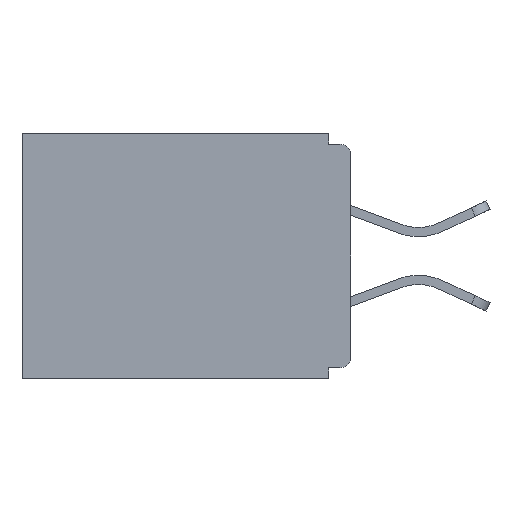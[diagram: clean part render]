
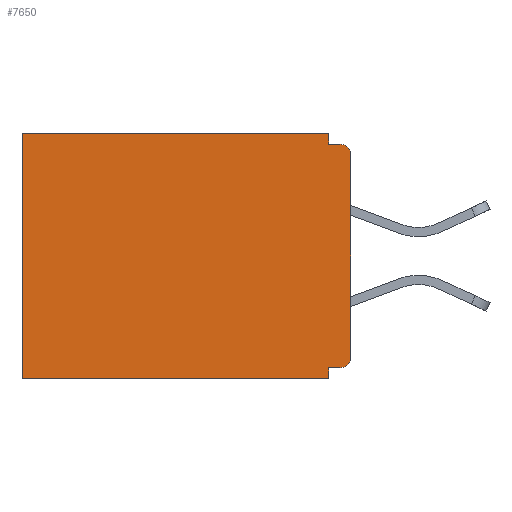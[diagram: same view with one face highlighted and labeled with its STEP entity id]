
A CAD part, left-side view. The second image highlights one B-rep face of the part: STEP entity #7650.
In plain terms, the highlighted planar face has unit normal (-1, 0, 0).
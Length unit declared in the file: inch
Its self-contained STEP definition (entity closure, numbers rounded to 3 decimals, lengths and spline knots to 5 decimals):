
#247 = EDGE_CURVE ( 'NONE', #10702, #9965, #11336, .T. ) ;
#285 = CIRCLE ( 'NONE', #10075, 0.015 ) ;
#392 = ORIENTED_EDGE ( 'NONE', *, *, #9194, .T. ) ;
#586 = VECTOR ( 'NONE', #7604, 39.37008 ) ;
#631 = VERTEX_POINT ( 'NONE', #12298 ) ;
#679 = DIRECTION ( 'NONE',  ( -1., 0., 0. ) ) ;
#1285 = CARTESIAN_POINT ( 'NONE',  ( 0.298, 0., 0. ) ) ;
#1431 = VERTEX_POINT ( 'NONE', #9696 ) ;
#1735 = CARTESIAN_POINT ( 'NONE',  ( 0.298, 0.031, -0.343 ) ) ;
#1775 = VECTOR ( 'NONE', #13323, 39.37008 ) ;
#1969 = PLANE ( 'NONE',  #9557 ) ;
#1972 = DIRECTION ( 'NONE',  ( 0., 0., -1. ) ) ;
#2337 = LINE ( 'NONE', #13573, #7540 ) ;
#2440 = ORIENTED_EDGE ( 'NONE', *, *, #2821, .F. ) ;
#2572 = LINE ( 'NONE', #5006, #1775 ) ;
#2622 = CARTESIAN_POINT ( 'NONE',  ( 0.298, 0., -0.343 ) ) ;
#2690 = DIRECTION ( 'NONE',  ( 0., 1., 0. ) ) ;
#2805 = ORIENTED_EDGE ( 'NONE', *, *, #12320, .T. ) ;
#2821 = EDGE_CURVE ( 'NONE', #631, #3070, #9476, .T. ) ;
#2861 = CARTESIAN_POINT ( 'NONE',  ( 0.298, 0.46, -0.343 ) ) ;
#2916 = CARTESIAN_POINT ( 'NONE',  ( 0.298, 0.031, -0.328 ) ) ;
#3070 = VERTEX_POINT ( 'NONE', #5585 ) ;
#3542 = EDGE_CURVE ( 'NONE', #10702, #631, #9281, .T. ) ;
#3596 = ORIENTED_EDGE ( 'NONE', *, *, #13413, .F. ) ;
#3681 = LINE ( 'NONE', #10999, #7186 ) ;
#3706 = VECTOR ( 'NONE', #7834, 39.37008 ) ;
#3944 = DIRECTION ( 'NONE',  ( 0., -1., 0. ) ) ;
#4145 = VECTOR ( 'NONE', #3944, 39.37008 ) ;
#4305 = DIRECTION ( 'NONE',  ( 0., 0., -1. ) ) ;
#4527 = EDGE_CURVE ( 'NONE', #7475, #8295, #2572, .T. ) ;
#4966 = ORIENTED_EDGE ( 'NONE', *, *, #7644, .T. ) ;
#5006 = CARTESIAN_POINT ( 'NONE',  ( 0.298, 0.031, -0.343 ) ) ;
#5582 = ORIENTED_EDGE ( 'NONE', *, *, #7792, .F. ) ;
#5585 = CARTESIAN_POINT ( 'NONE',  ( 0.298, 0.015, -0.015 ) ) ;
#5811 = CIRCLE ( 'NONE', #7746, 0.015 ) ;
#6187 = CARTESIAN_POINT ( 'NONE',  ( 0.298, 0., -0.015 ) ) ;
#6189 = CARTESIAN_POINT ( 'NONE',  ( 0.298, 0., -0.03 ) ) ;
#6312 = CARTESIAN_POINT ( 'NONE',  ( 0.298, 0.015, -0.313 ) ) ;
#6407 = CARTESIAN_POINT ( 'NONE',  ( 0.298, 0.031, -0.343 ) ) ;
#6782 = DIRECTION ( 'NONE',  ( 0., 1., 0. ) ) ;
#6968 = EDGE_LOOP ( 'NONE', ( #392, #2440, #8042, #12238, #4966, #9730, #11913, #5582, #2805, #3596 ) ) ;
#7186 = VECTOR ( 'NONE', #2690, 39.37008 ) ;
#7320 = CARTESIAN_POINT ( 'NONE',  ( 0.298, 0., 0. ) ) ;
#7475 = VERTEX_POINT ( 'NONE', #2916 ) ;
#7540 = VECTOR ( 'NONE', #8351, 39.37008 ) ;
#7604 = DIRECTION ( 'NONE',  ( 0., 0., -1. ) ) ;
#7644 = EDGE_CURVE ( 'NONE', #9965, #11980, #2337, .T. ) ;
#7650 = ADVANCED_FACE ( 'NONE', ( #13314 ), #1969, .F. ) ;
#7746 = AXIS2_PLACEMENT_3D ( 'NONE', #8178, #679, #10113 ) ;
#7792 = EDGE_CURVE ( 'NONE', #1431, #7475, #3681, .T. ) ;
#7834 = DIRECTION ( 'NONE',  ( 0., 1., 0. ) ) ;
#8042 = ORIENTED_EDGE ( 'NONE', *, *, #3542, .F. ) ;
#8178 = CARTESIAN_POINT ( 'NONE',  ( 0.298, 0.015, -0.03 ) ) ;
#8295 = VERTEX_POINT ( 'NONE', #1735 ) ;
#8351 = DIRECTION ( 'NONE',  ( 0., 0., -1. ) ) ;
#8401 = DIRECTION ( 'NONE',  ( 1., 0., 0. ) ) ;
#8441 = VERTEX_POINT ( 'NONE', #10213 ) ;
#8552 = CARTESIAN_POINT ( 'NONE',  ( 0.298, 0.46, 0. ) ) ;
#9027 = LINE ( 'NONE', #2622, #11504 ) ;
#9059 = LINE ( 'NONE', #1285, #586 ) ;
#9194 = EDGE_CURVE ( 'NONE', #10132, #3070, #5811, .T. ) ;
#9281 = LINE ( 'NONE', #6407, #13210 ) ;
#9395 = DIRECTION ( 'NONE',  ( 0., 0., -1. ) ) ;
#9476 = LINE ( 'NONE', #6187, #4145 ) ;
#9525 = DIRECTION ( 'NONE',  ( -1., 0., 0. ) ) ;
#9557 = AXIS2_PLACEMENT_3D ( 'NONE', #7320, #8401, #9395 ) ;
#9659 = CARTESIAN_POINT ( 'NONE',  ( 0.298, 0.031, 0. ) ) ;
#9696 = CARTESIAN_POINT ( 'NONE',  ( 0.298, 0.015, -0.328 ) ) ;
#9730 = ORIENTED_EDGE ( 'NONE', *, *, #12888, .F. ) ;
#9965 = VERTEX_POINT ( 'NONE', #8552 ) ;
#10075 = AXIS2_PLACEMENT_3D ( 'NONE', #6312, #9525, #1972 ) ;
#10113 = DIRECTION ( 'NONE',  ( 0., 0., -1. ) ) ;
#10132 = VERTEX_POINT ( 'NONE', #6189 ) ;
#10213 = CARTESIAN_POINT ( 'NONE',  ( 0.298, 0., -0.313 ) ) ;
#10302 = CARTESIAN_POINT ( 'NONE',  ( 0.298, 0., 0. ) ) ;
#10702 = VERTEX_POINT ( 'NONE', #9659 ) ;
#10999 = CARTESIAN_POINT ( 'NONE',  ( 0.298, 0., -0.328 ) ) ;
#11336 = LINE ( 'NONE', #10302, #3706 ) ;
#11504 = VECTOR ( 'NONE', #6782, 39.37008 ) ;
#11913 = ORIENTED_EDGE ( 'NONE', *, *, #4527, .F. ) ;
#11980 = VERTEX_POINT ( 'NONE', #2861 ) ;
#12238 = ORIENTED_EDGE ( 'NONE', *, *, #247, .T. ) ;
#12298 = CARTESIAN_POINT ( 'NONE',  ( 0.298, 0.031, -0.015 ) ) ;
#12320 = EDGE_CURVE ( 'NONE', #1431, #8441, #285, .T. ) ;
#12888 = EDGE_CURVE ( 'NONE', #8295, #11980, #9027, .T. ) ;
#13210 = VECTOR ( 'NONE', #4305, 39.37008 ) ;
#13314 = FACE_OUTER_BOUND ( 'NONE', #6968, .T. ) ;
#13323 = DIRECTION ( 'NONE',  ( 0., 0., -1. ) ) ;
#13413 = EDGE_CURVE ( 'NONE', #10132, #8441, #9059, .T. ) ;
#13573 = CARTESIAN_POINT ( 'NONE',  ( 0.298, 0.46, 0. ) ) ;
